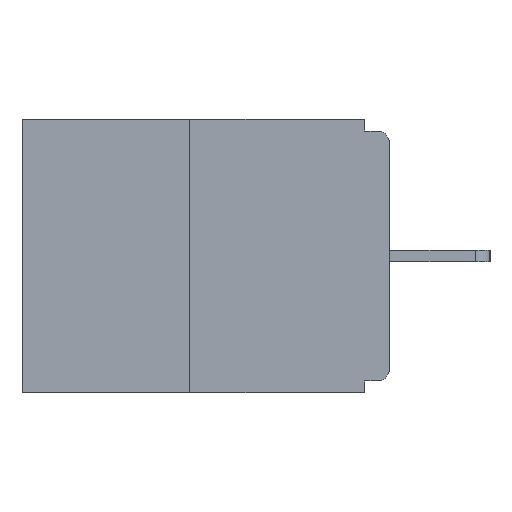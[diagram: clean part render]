
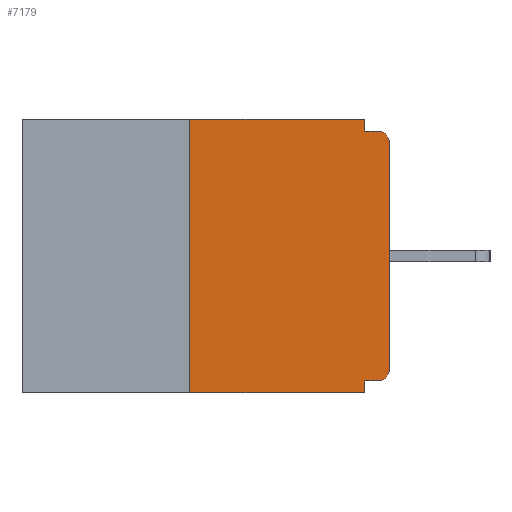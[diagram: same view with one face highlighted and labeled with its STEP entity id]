
A CAD part, left-side view. The second image highlights one B-rep face of the part: STEP entity #7179.
In plain terms, the highlighted planar face has unit normal (-1, 0, 0).
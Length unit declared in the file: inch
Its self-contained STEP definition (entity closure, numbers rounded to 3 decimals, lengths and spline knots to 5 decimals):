
#149 = VECTOR ( 'NONE', #9293, 39.37008 ) ;
#194 = DIRECTION ( 'NONE',  ( 0., 0., -1. ) ) ;
#431 = DIRECTION ( 'NONE',  ( 0., 0., 1. ) ) ;
#486 = FACE_OUTER_BOUND ( 'NONE', #4699, .T. ) ;
#534 = VECTOR ( 'NONE', #1748, 39.37008 ) ;
#636 = ORIENTED_EDGE ( 'NONE', *, *, #3489, .F. ) ;
#679 = ORIENTED_EDGE ( 'NONE', *, *, #8805, .T. ) ;
#770 = ORIENTED_EDGE ( 'NONE', *, *, #4632, .F. ) ;
#865 = VERTEX_POINT ( 'NONE', #5240 ) ;
#944 = CARTESIAN_POINT ( 'NONE',  ( 0., 0.25, 0. ) ) ;
#960 = ORIENTED_EDGE ( 'NONE', *, *, #7105, .F. ) ;
#1748 = DIRECTION ( 'NONE',  ( 0., 0., 1. ) ) ;
#1764 = VECTOR ( 'NONE', #194, 39.37008 ) ;
#1883 = DIRECTION ( 'NONE',  ( -1., 0., 0. ) ) ;
#2195 = EDGE_CURVE ( 'NONE', #5095, #6359, #6495, .T. ) ;
#2514 = VERTEX_POINT ( 'NONE', #4433 ) ;
#2714 = VERTEX_POINT ( 'NONE', #7387 ) ;
#2849 = LINE ( 'NONE', #4694, #2933 ) ;
#2871 = DIRECTION ( 'NONE',  ( 1., 0., 0. ) ) ;
#2883 = CARTESIAN_POINT ( 'NONE',  ( 0., 0.015, -0.03 ) ) ;
#2915 = CARTESIAN_POINT ( 'NONE',  ( 0., 0., 0. ) ) ;
#2925 = EDGE_CURVE ( 'NONE', #2714, #5855, #7193, .T. ) ;
#2928 = DIRECTION ( 'NONE',  ( 0., 0., -1. ) ) ;
#2933 = VECTOR ( 'NONE', #6372, 39.37008 ) ;
#3007 = AXIS2_PLACEMENT_3D ( 'NONE', #2883, #1883, #3740 ) ;
#3021 = LINE ( 'NONE', #3771, #149 ) ;
#3379 = DIRECTION ( 'NONE',  ( 0., 0., -1. ) ) ;
#3489 = EDGE_CURVE ( 'NONE', #5095, #3900, #2849, .T. ) ;
#3653 = LINE ( 'NONE', #7185, #1764 ) ;
#3740 = DIRECTION ( 'NONE',  ( 0., 0., -1. ) ) ;
#3771 = CARTESIAN_POINT ( 'NONE',  ( 0., 0.46, -0.343 ) ) ;
#3828 = CARTESIAN_POINT ( 'NONE',  ( 0., 0.015, -0.015 ) ) ;
#3900 = VERTEX_POINT ( 'NONE', #7505 ) ;
#4016 = CARTESIAN_POINT ( 'NONE',  ( 0., 0., -0.015 ) ) ;
#4433 = CARTESIAN_POINT ( 'NONE',  ( 0., 0.031, -0.015 ) ) ;
#4558 = VERTEX_POINT ( 'NONE', #5215 ) ;
#4601 = CARTESIAN_POINT ( 'NONE',  ( 0., 0.46, 0. ) ) ;
#4632 = EDGE_CURVE ( 'NONE', #4558, #2514, #3653, .T. ) ;
#4694 = CARTESIAN_POINT ( 'NONE',  ( 0., 0., -0.328 ) ) ;
#4699 = EDGE_LOOP ( 'NONE', ( #7381, #9466, #9772, #7009, #636, #5019, #679, #5436, #960, #770 ) ) ;
#4816 = LINE ( 'NONE', #2915, #6947 ) ;
#4911 = DIRECTION ( 'NONE',  ( 0., 0., -1. ) ) ;
#5019 = ORIENTED_EDGE ( 'NONE', *, *, #2195, .T. ) ;
#5039 = CARTESIAN_POINT ( 'NONE',  ( 0., 0., -0.03 ) ) ;
#5095 = VERTEX_POINT ( 'NONE', #7827 ) ;
#5174 = CARTESIAN_POINT ( 'NONE',  ( 0., 0.25, 0. ) ) ;
#5215 = CARTESIAN_POINT ( 'NONE',  ( 0., 0.031, 0. ) ) ;
#5240 = CARTESIAN_POINT ( 'NONE',  ( 0., 0.031, -0.343 ) ) ;
#5428 = VECTOR ( 'NONE', #8537, 39.37008 ) ;
#5436 = ORIENTED_EDGE ( 'NONE', *, *, #11278, .T. ) ;
#5544 = CARTESIAN_POINT ( 'NONE',  ( 0., 0.015, -0.313 ) ) ;
#5576 = LINE ( 'NONE', #4016, #5428 ) ;
#5668 = EDGE_CURVE ( 'NONE', #3900, #865, #11325, .T. ) ;
#5855 = VERTEX_POINT ( 'NONE', #944 ) ;
#6048 = VERTEX_POINT ( 'NONE', #5039 ) ;
#6358 = VECTOR ( 'NONE', #3379, 39.37008 ) ;
#6359 = VERTEX_POINT ( 'NONE', #9398 ) ;
#6372 = DIRECTION ( 'NONE',  ( 0., 1., 0. ) ) ;
#6495 = CIRCLE ( 'NONE', #7437, 0.015 ) ;
#6666 = PLANE ( 'NONE',  #10268 ) ;
#6947 = VECTOR ( 'NONE', #431, 39.37008 ) ;
#7009 = ORIENTED_EDGE ( 'NONE', *, *, #5668, .F. ) ;
#7105 = EDGE_CURVE ( 'NONE', #2514, #10415, #5576, .T. ) ;
#7179 = ADVANCED_FACE ( 'NONE', ( #486 ), #6666, .F. ) ;
#7185 = CARTESIAN_POINT ( 'NONE',  ( 0., 0.031, 0. ) ) ;
#7193 = LINE ( 'NONE', #5174, #534 ) ;
#7381 = ORIENTED_EDGE ( 'NONE', *, *, #9455, .F. ) ;
#7387 = CARTESIAN_POINT ( 'NONE',  ( 0., 0.25, -0.343 ) ) ;
#7437 = AXIS2_PLACEMENT_3D ( 'NONE', #5544, #10876, #4911 ) ;
#7505 = CARTESIAN_POINT ( 'NONE',  ( 0., 0.031, -0.328 ) ) ;
#7523 = VECTOR ( 'NONE', #8909, 39.37008 ) ;
#7820 = CIRCLE ( 'NONE', #3007, 0.015 ) ;
#7827 = CARTESIAN_POINT ( 'NONE',  ( 0., 0.015, -0.328 ) ) ;
#8537 = DIRECTION ( 'NONE',  ( 0., -1., 0. ) ) ;
#8805 = EDGE_CURVE ( 'NONE', #6359, #6048, #4816, .T. ) ;
#8909 = DIRECTION ( 'NONE',  ( 0., -1., 0. ) ) ;
#9293 = DIRECTION ( 'NONE',  ( 0., -1., 0. ) ) ;
#9398 = CARTESIAN_POINT ( 'NONE',  ( 0., 0., -0.313 ) ) ;
#9428 = CARTESIAN_POINT ( 'NONE',  ( 0., 0.031, -0.343 ) ) ;
#9455 = EDGE_CURVE ( 'NONE', #5855, #4558, #9776, .T. ) ;
#9466 = ORIENTED_EDGE ( 'NONE', *, *, #2925, .F. ) ;
#9772 = ORIENTED_EDGE ( 'NONE', *, *, #10440, .T. ) ;
#9776 = LINE ( 'NONE', #4601, #7523 ) ;
#10216 = CARTESIAN_POINT ( 'NONE',  ( 0., 0.46, 0. ) ) ;
#10268 = AXIS2_PLACEMENT_3D ( 'NONE', #10216, #2871, #2928 ) ;
#10415 = VERTEX_POINT ( 'NONE', #3828 ) ;
#10440 = EDGE_CURVE ( 'NONE', #2714, #865, #3021, .T. ) ;
#10876 = DIRECTION ( 'NONE',  ( -1., 0., 0. ) ) ;
#11278 = EDGE_CURVE ( 'NONE', #6048, #10415, #7820, .T. ) ;
#11325 = LINE ( 'NONE', #9428, #6358 ) ;
